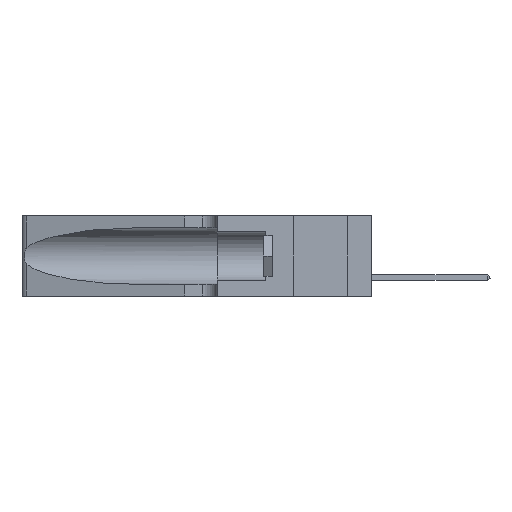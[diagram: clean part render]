
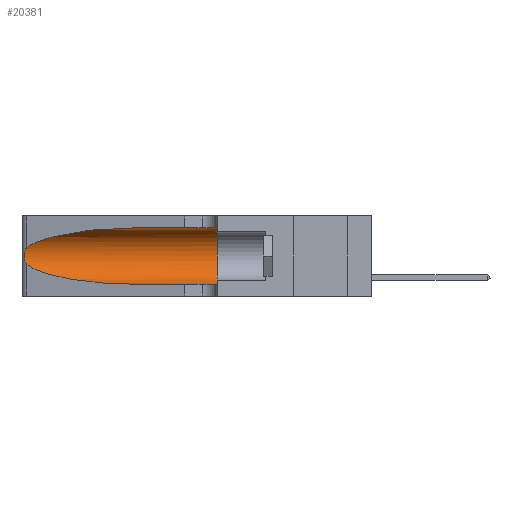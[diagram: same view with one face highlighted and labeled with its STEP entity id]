
A CAD part, left-side view. The second image highlights one B-rep face of the part: STEP entity #20381.
In plain terms, the highlighted cylindrical face has radius 3.308 mm (diameter 6.617 mm), a partial arc.
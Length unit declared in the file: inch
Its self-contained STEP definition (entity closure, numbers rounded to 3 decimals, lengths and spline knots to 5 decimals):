
#115 = CARTESIAN_POINT ( 'NONE',  ( 0.1305, 0.35, 0.05475 ) ) ;
#402 = CARTESIAN_POINT ( 'NONE',  ( 0.26017, 1.23833, 0.17102 ) ) ;
#1027 = DIRECTION ( 'NONE',  ( 0., 1., 0. ) ) ;
#2422 = CARTESIAN_POINT ( 'NONE',  ( 0.25787, 1.23484, 0.2124 ) ) ;
#2592 = EDGE_CURVE ( 'NONE', #27640, #17322, #21115, .T. ) ;
#2704 = ORIENTED_EDGE ( 'NONE', *, *, #10145, .F. ) ;
#2954 = VERTEX_POINT ( 'NONE', #115 ) ;
#3002 = CARTESIAN_POINT ( 'NONE',  ( 0.2373, 1.15595, 0.08982 ) ) ;
#3305 = DIRECTION ( 'NONE',  ( 0., -1., 0. ) ) ;
#3315 = ORIENTED_EDGE ( 'NONE', *, *, #5583, .T. ) ;
#3975 = EDGE_LOOP ( 'NONE', ( #3315, #17618, #15816, #26001, #25872, #2704 ) ) ;
#4204 = EDGE_CURVE ( 'NONE', #17322, #2954, #26010, .T. ) ;
#4402 = VECTOR ( 'NONE', #31844, 39.37008 ) ;
#4769 = CARTESIAN_POINT ( 'NONE',  ( 0.25555, 1.22994, 0.2215 ) ) ;
#4860 = CARTESIAN_POINT ( 'NONE',  ( 0.1305, 1.61858, 0.185 ) ) ;
#5583 = EDGE_CURVE ( 'NONE', #6728, #17069, #7235, .T. ) ;
#5967 = DIRECTION ( 'NONE',  ( 0., 0., 1. ) ) ;
#6458 = EDGE_CURVE ( 'NONE', #17069, #27640, #23521, .T. ) ;
#6728 = VERTEX_POINT ( 'NONE', #28721 ) ;
#6808 = FACE_OUTER_BOUND ( 'NONE', #3975, .T. ) ;
#7021 = DIRECTION ( 'NONE',  ( 0., -1., 0. ) ) ;
#7235 =( BOUNDED_CURVE ( )  B_SPLINE_CURVE ( 3, ( #22192, #9918, #14996, #31961 ),
 .UNSPECIFIED., .F., .F. ) 
 B_SPLINE_CURVE_WITH_KNOTS ( ( 4, 4 ),
 ( 1.5708, 2.84003 ),
 .UNSPECIFIED. ) 
 CURVE ( )  GEOMETRIC_REPRESENTATION_ITEM ( )  RATIONAL_B_SPLINE_CURVE ( ( 1., 0.87, 0.87, 1. ) ) 
 REPRESENTATION_ITEM ( '' )  );
#7248 = CARTESIAN_POINT ( 'NONE',  ( 0.25639, 1.23184, 0.21858 ) ) ;
#7786 = EDGE_CURVE ( 'NONE', #11065, #2954, #30799, .T. ) ;
#8142 = CARTESIAN_POINT ( 'NONE',  ( 0.26075, 1.23896, 0.19203 ) ) ;
#9918 = CARTESIAN_POINT ( 'NONE',  ( 0.18966, 0.96281, 0.31525 ) ) ;
#10145 = EDGE_CURVE ( 'NONE', #6728, #11065, #11733, .T. ) ;
#11065 = VERTEX_POINT ( 'NONE', #22245 ) ;
#11733 = LINE ( 'NONE', #17390, #4402 ) ;
#13284 = CARTESIAN_POINT ( 'NONE',  ( 0.1305, 0.35, 0.185 ) ) ;
#14996 = CARTESIAN_POINT ( 'NONE',  ( 0.2373, 1.15595, 0.28018 ) ) ;
#15394 = CARTESIAN_POINT ( 'NONE',  ( 0.25854, 1.2359, 0.20912 ) ) ;
#15816 = ORIENTED_EDGE ( 'NONE', *, *, #2592, .T. ) ;
#17069 = VERTEX_POINT ( 'NONE', #20671 ) ;
#17322 = VERTEX_POINT ( 'NONE', #18175 ) ;
#17390 = CARTESIAN_POINT ( 'NONE',  ( 0.1305, 1.61858, 0.31525 ) ) ;
#17574 = CARTESIAN_POINT ( 'NONE',  ( 0.25856, 1.23593, 0.16098 ) ) ;
#17618 = ORIENTED_EDGE ( 'NONE', *, *, #6458, .T. ) ;
#17679 = CARTESIAN_POINT ( 'NONE',  ( 0.26075, 1.23896, 0.178 ) ) ;
#17799 = CARTESIAN_POINT ( 'NONE',  ( 0.25639, 1.23186, 0.15144 ) ) ;
#18175 = CARTESIAN_POINT ( 'NONE',  ( 0.1305, 0.72297, 0.05475 ) ) ;
#18467 = CARTESIAN_POINT ( 'NONE',  ( 0.25487, 1.22718, 0.14631 ) ) ;
#19614 = CARTESIAN_POINT ( 'NONE',  ( 0.25487, 1.22718, 0.22369 ) ) ;
#19632 = CYLINDRICAL_SURFACE ( 'NONE', #32032, 0.13025 ) ;
#20381 = ADVANCED_FACE ( 'NONE', ( #6808 ), #19632, .F. ) ;
#20507 = CARTESIAN_POINT ( 'NONE',  ( 0.25789, 1.23486, 0.15765 ) ) ;
#20671 = CARTESIAN_POINT ( 'NONE',  ( 0.25487, 1.22718, 0.22369 ) ) ;
#21115 =( BOUNDED_CURVE ( )  B_SPLINE_CURVE ( 3, ( #26022, #3002, #30746, #25909 ),
 .UNSPECIFIED., .F., .F. ) 
 B_SPLINE_CURVE_WITH_KNOTS ( ( 4, 4 ),
 ( 3.44316, 4.71239 ),
 .UNSPECIFIED. ) 
 CURVE ( )  GEOMETRIC_REPRESENTATION_ITEM ( )  RATIONAL_B_SPLINE_CURVE ( ( 1., 0.87, 0.87, 1. ) ) 
 REPRESENTATION_ITEM ( '' )  );
#22089 = DIRECTION ( 'NONE',  ( 0., 0., -1. ) ) ;
#22192 = CARTESIAN_POINT ( 'NONE',  ( 0.1305, 0.72297, 0.31525 ) ) ;
#22245 = CARTESIAN_POINT ( 'NONE',  ( 0.1305, 0.35, 0.31525 ) ) ;
#22904 = CARTESIAN_POINT ( 'NONE',  ( 0.25487, 1.22718, 0.14631 ) ) ;
#23309 = VECTOR ( 'NONE', #3305, 39.37008 ) ;
#23521 = B_SPLINE_CURVE_WITH_KNOTS ( 'NONE', 3,
 ( #19614, #4769, #7248, #2422, #15394, #27831, #8142, #17679, #402, #17574, #20507, #17799, #25257, #22904 ),
 .UNSPECIFIED., .F., .F.,
 ( 4, 2, 2, 2, 2, 2, 4 ),
 ( 0., 0.00027, 0.00053, 0.00107, 0.0016, 0.00187, 0.00214 ),
 .UNSPECIFIED. ) ;
#25257 = CARTESIAN_POINT ( 'NONE',  ( 0.25555, 1.22993, 0.14849 ) ) ;
#25872 = ORIENTED_EDGE ( 'NONE', *, *, #7786, .F. ) ;
#25909 = CARTESIAN_POINT ( 'NONE',  ( 0.1305, 0.72297, 0.05475 ) ) ;
#26001 = ORIENTED_EDGE ( 'NONE', *, *, #4204, .T. ) ;
#26010 = LINE ( 'NONE', #27564, #23309 ) ;
#26022 = CARTESIAN_POINT ( 'NONE',  ( 0.25487, 1.22718, 0.14631 ) ) ;
#27249 = AXIS2_PLACEMENT_3D ( 'NONE', #13284, #1027, #5967 ) ;
#27564 = CARTESIAN_POINT ( 'NONE',  ( 0.1305, 1.61858, 0.05475 ) ) ;
#27640 = VERTEX_POINT ( 'NONE', #18467 ) ;
#27831 = CARTESIAN_POINT ( 'NONE',  ( 0.26018, 1.23835, 0.19895 ) ) ;
#28721 = CARTESIAN_POINT ( 'NONE',  ( 0.1305, 0.72297, 0.31525 ) ) ;
#30746 = CARTESIAN_POINT ( 'NONE',  ( 0.18966, 0.96281, 0.05475 ) ) ;
#30799 = CIRCLE ( 'NONE', #27249, 0.13025 ) ;
#31844 = DIRECTION ( 'NONE',  ( 0., -1., 0. ) ) ;
#31961 = CARTESIAN_POINT ( 'NONE',  ( 0.25487, 1.22718, 0.22369 ) ) ;
#32032 = AXIS2_PLACEMENT_3D ( 'NONE', #4860, #7021, #22089 ) ;
